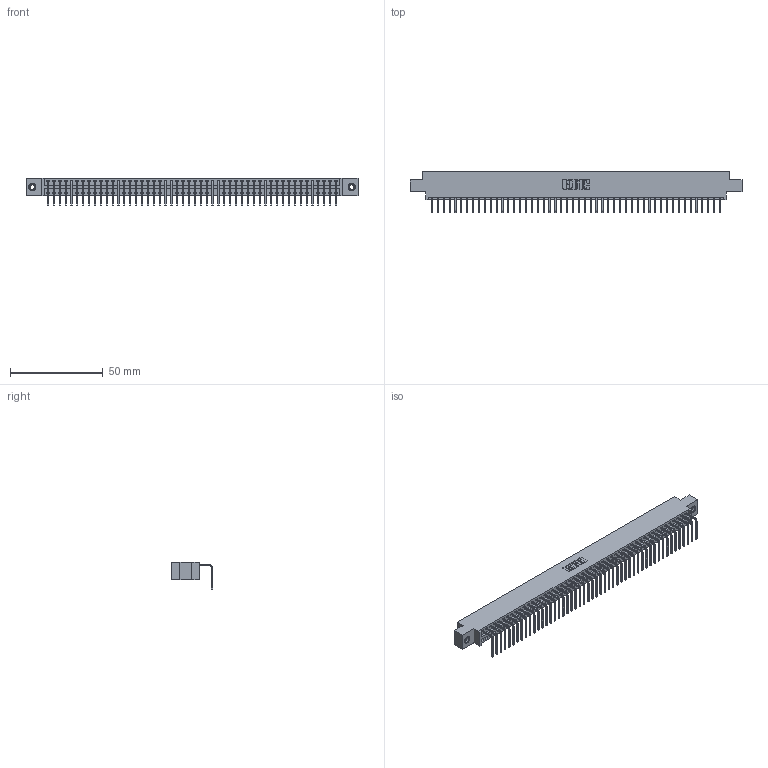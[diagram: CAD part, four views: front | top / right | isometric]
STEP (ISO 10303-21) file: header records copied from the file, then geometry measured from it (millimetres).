
FILE_DESCRIPTION (( 'STEP AP203' ), '1' );
FILE_NAME ('346-050-558-607.STEP', '2022-05-10T04:09:08', ( '' ), ( '' ), 'SwSTEP 2.0', 'SolidWorks 2020', '' );
FILE_SCHEMA (( 'CONFIG_CONTROL_DESIGN' ));
Length unit declared in the file: inch
Products named in the file (4): 345-250-001_345-250-005-103; 346-050-558-607; 346 Part_0.170 Offset - 0.156 Dia-TI; 345-292-001_558 Tail - 2
Assembly tree (53 placements, depth 2):
  346-050-558-607
    346 Part_0.170 Offset - 0.156 Dia-TI
    345-292-001_558 Tail - 2  x50
    345-250-001_345-250-005-103  x2
Bounding box: 179.32 x 22.16 x 14.73 mm (x, y, z)
Volume: 830.8 mm3; surface area: 22709.8 mm2
Topology: 52 solids, 53 shells, 3178 faces, 9577 edges, 6310 vertices
Faces by surface type: plane 2204, cylinder 958, cone 12, torus 4
Entity records: 31356 total; most frequent: CARTESIAN_POINT 5357, ORIENTED_EDGE 5334, DIRECTION 4741, EDGE_CURVE 2667, LINE 2315, VECTOR 2315, VERTEX_POINT 1772, AXIS2_PLACEMENT_3D 1213
